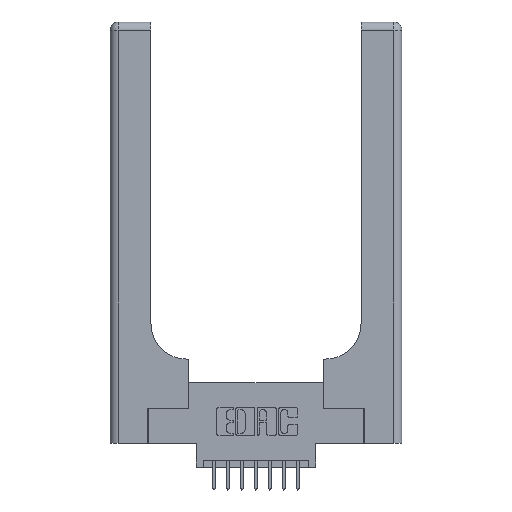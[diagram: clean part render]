
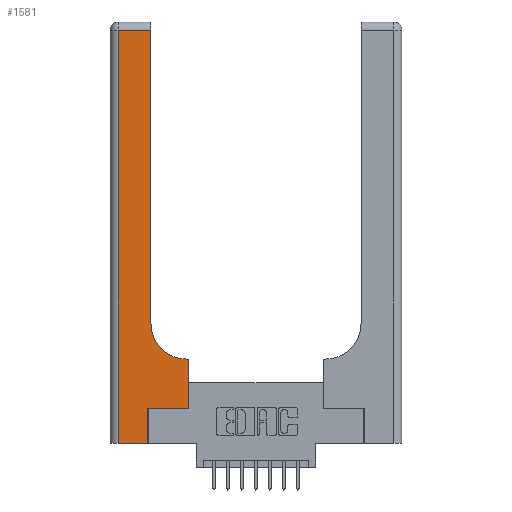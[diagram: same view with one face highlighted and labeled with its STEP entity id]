
A CAD part, top view. The second image highlights one B-rep face of the part: STEP entity #1581.
In plain terms, the highlighted planar face has unit normal (0, 0, 1).
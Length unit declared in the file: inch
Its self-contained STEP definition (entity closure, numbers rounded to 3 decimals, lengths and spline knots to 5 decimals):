
#220 = VECTOR ( 'NONE', #3271, 39.37008 ) ;
#330 = CARTESIAN_POINT ( 'NONE',  ( 0.269, 0., 0.37 ) ) ;
#430 = LINE ( 'NONE', #12113, #6630 ) ;
#610 = LINE ( 'NONE', #10214, #6787 ) ;
#672 = EDGE_CURVE ( 'NONE', #14582, #7207, #430, .T. ) ;
#905 = EDGE_CURVE ( 'NONE', #7498, #3950, #3958, .T. ) ;
#961 = LINE ( 'NONE', #9591, #13475 ) ;
#1086 = DIRECTION ( 'NONE',  ( 0., 1., 0. ) ) ;
#1196 = CARTESIAN_POINT ( 'NONE',  ( 0., 0., 0.37 ) ) ;
#1200 = ORIENTED_EDGE ( 'NONE', *, *, #2361, .T. ) ;
#1408 = EDGE_CURVE ( 'NONE', #14853, #7498, #610, .T. ) ;
#1436 = AXIS2_PLACEMENT_3D ( 'NONE', #3192, #11671, #4467 ) ;
#1581 = ADVANCED_FACE ( 'NONE', ( #10918 ), #7692, .F. ) ;
#1680 = ORIENTED_EDGE ( 'NONE', *, *, #1408, .T. ) ;
#1774 = CARTESIAN_POINT ( 'NONE',  ( 0.2915, 2.94, 0.37 ) ) ;
#2361 = EDGE_CURVE ( 'NONE', #12658, #11660, #961, .T. ) ;
#2569 = AXIS2_PLACEMENT_3D ( 'NONE', #7639, #7617, #7596 ) ;
#2666 = ORIENTED_EDGE ( 'NONE', *, *, #672, .T. ) ;
#2752 = EDGE_CURVE ( 'NONE', #6362, #12658, #12399, .T. ) ;
#2984 = ORIENTED_EDGE ( 'NONE', *, *, #11019, .T. ) ;
#3192 = CARTESIAN_POINT ( 'NONE',  ( 0.5415, 0.85, 0.37 ) ) ;
#3271 = DIRECTION ( 'NONE',  ( 1., 0., 0. ) ) ;
#3417 = CARTESIAN_POINT ( 'NONE',  ( 0.269, 0.25, 0.37 ) ) ;
#3782 = LINE ( 'NONE', #6022, #12637 ) ;
#3831 = EDGE_LOOP ( 'NONE', ( #15400, #11655, #1200, #2984, #1680, #6829, #14671, #2666, #7983 ) ) ;
#3950 = VERTEX_POINT ( 'NONE', #8025 ) ;
#3958 = LINE ( 'NONE', #3417, #220 ) ;
#4030 = VECTOR ( 'NONE', #1086, 39.37008 ) ;
#4467 = DIRECTION ( 'NONE',  ( 1., 0., 0. ) ) ;
#4596 = CARTESIAN_POINT ( 'NONE',  ( 0.5585, 0.25, 0.37 ) ) ;
#4813 = LINE ( 'NONE', #4596, #4030 ) ;
#6022 = CARTESIAN_POINT ( 'NONE',  ( 0.2915, 3., 0.37 ) ) ;
#6023 = DIRECTION ( 'NONE',  ( 0., -1., 0. ) ) ;
#6113 = CARTESIAN_POINT ( 'NONE',  ( 0.06, 0., 0.37 ) ) ;
#6362 = VERTEX_POINT ( 'NONE', #1774 ) ;
#6418 = EDGE_CURVE ( 'NONE', #7207, #11965, #10662, .T. ) ;
#6630 = VECTOR ( 'NONE', #12026, 39.37008 ) ;
#6787 = VECTOR ( 'NONE', #10530, 39.37008 ) ;
#6829 = ORIENTED_EDGE ( 'NONE', *, *, #905, .T. ) ;
#7207 = VERTEX_POINT ( 'NONE', #14519 ) ;
#7222 = DIRECTION ( 'NONE',  ( 1., 0., 0. ) ) ;
#7498 = VERTEX_POINT ( 'NONE', #7913 ) ;
#7596 = DIRECTION ( 'NONE',  ( -1., 0., 0. ) ) ;
#7617 = DIRECTION ( 'NONE',  ( 0., 0., -1. ) ) ;
#7639 = CARTESIAN_POINT ( 'NONE',  ( 0., 3., 0.37 ) ) ;
#7692 = PLANE ( 'NONE',  #2569 ) ;
#7909 = EDGE_CURVE ( 'NONE', #3950, #14582, #4813, .T. ) ;
#7913 = CARTESIAN_POINT ( 'NONE',  ( 0.269, 0.25, 0.37 ) ) ;
#7983 = ORIENTED_EDGE ( 'NONE', *, *, #6418, .T. ) ;
#8025 = CARTESIAN_POINT ( 'NONE',  ( 0.5585, 0.25, 0.37 ) ) ;
#8163 = DIRECTION ( 'NONE',  ( -1., 0., 0. ) ) ;
#9209 = VECTOR ( 'NONE', #8163, 39.37008 ) ;
#9492 = CARTESIAN_POINT ( 'NONE',  ( 0.06, 2.94, 0.37 ) ) ;
#9591 = CARTESIAN_POINT ( 'NONE',  ( 0.06, 3., 0.37 ) ) ;
#9616 = EDGE_CURVE ( 'NONE', #11965, #6362, #3782, .T. ) ;
#10214 = CARTESIAN_POINT ( 'NONE',  ( 0.269, 0., 0.37 ) ) ;
#10530 = DIRECTION ( 'NONE',  ( 0., 1., 0. ) ) ;
#10662 = CIRCLE ( 'NONE', #1436, 0.25 ) ;
#10918 = FACE_OUTER_BOUND ( 'NONE', #3831, .T. ) ;
#11019 = EDGE_CURVE ( 'NONE', #11660, #14853, #11615, .T. ) ;
#11402 = CARTESIAN_POINT ( 'NONE',  ( 0.2915, 0.85, 0.37 ) ) ;
#11615 = LINE ( 'NONE', #1196, #11980 ) ;
#11655 = ORIENTED_EDGE ( 'NONE', *, *, #2752, .T. ) ;
#11660 = VERTEX_POINT ( 'NONE', #6113 ) ;
#11671 = DIRECTION ( 'NONE',  ( 0., 0., -1. ) ) ;
#11965 = VERTEX_POINT ( 'NONE', #11402 ) ;
#11980 = VECTOR ( 'NONE', #7222, 39.37008 ) ;
#12026 = DIRECTION ( 'NONE',  ( -1., 0., 0. ) ) ;
#12113 = CARTESIAN_POINT ( 'NONE',  ( 0.2915, 0.6, 0.37 ) ) ;
#12399 = LINE ( 'NONE', #14082, #9209 ) ;
#12637 = VECTOR ( 'NONE', #15485, 39.37008 ) ;
#12658 = VERTEX_POINT ( 'NONE', #9492 ) ;
#13475 = VECTOR ( 'NONE', #6023, 39.37008 ) ;
#14082 = CARTESIAN_POINT ( 'NONE',  ( 0., 2.94, 0.37 ) ) ;
#14519 = CARTESIAN_POINT ( 'NONE',  ( 0.5415, 0.6, 0.37 ) ) ;
#14582 = VERTEX_POINT ( 'NONE', #15155 ) ;
#14671 = ORIENTED_EDGE ( 'NONE', *, *, #7909, .T. ) ;
#14853 = VERTEX_POINT ( 'NONE', #330 ) ;
#15155 = CARTESIAN_POINT ( 'NONE',  ( 0.5585, 0.6, 0.37 ) ) ;
#15400 = ORIENTED_EDGE ( 'NONE', *, *, #9616, .T. ) ;
#15485 = DIRECTION ( 'NONE',  ( 0., 1., 0. ) ) ;
